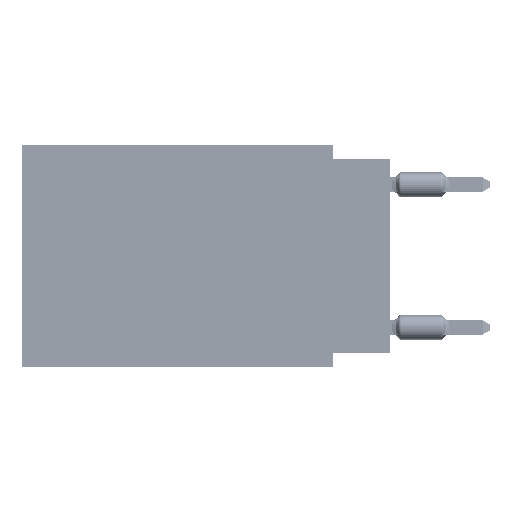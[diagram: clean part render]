
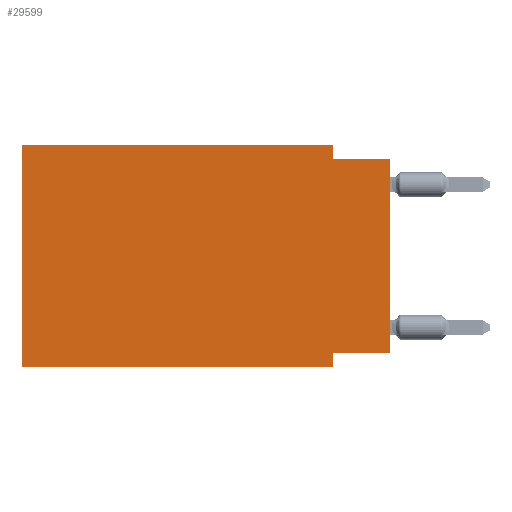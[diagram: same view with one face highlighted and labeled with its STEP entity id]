
A CAD part, left-side view. The second image highlights one B-rep face of the part: STEP entity #29599.
In plain terms, the highlighted planar face has unit normal (-1, 0, 0).
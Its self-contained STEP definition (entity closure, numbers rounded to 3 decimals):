
#4770 = CARTESIAN_POINT ( 'NONE',  ( 0., 16.383, 0. ) ) ;
#7644 = EDGE_CURVE ( 'NONE', #35480, #17729, #47735, .T. ) ;
#8155 = ORIENTED_EDGE ( 'NONE', *, *, #63120, .F. ) ;
#8812 = VERTEX_POINT ( 'NONE', #18402 ) ;
#9850 = LINE ( 'NONE', #53430, #20157 ) ;
#10892 = ORIENTED_EDGE ( 'NONE', *, *, #14784, .F. ) ;
#11123 = EDGE_CURVE ( 'NONE', #54508, #53946, #21433, .T. ) ;
#11404 = VERTEX_POINT ( 'NONE', #20290 ) ;
#12124 = VECTOR ( 'NONE', #36971, 1000. ) ;
#14080 = CARTESIAN_POINT ( 'NONE',  ( 0., 0., -0.635 ) ) ;
#14484 = VECTOR ( 'NONE', #26203, 1000. ) ;
#14494 = CARTESIAN_POINT ( 'NONE',  ( 0., 2.54, 0. ) ) ;
#14784 = EDGE_CURVE ( 'NONE', #8812, #11404, #59131, .T. ) ;
#14804 = EDGE_CURVE ( 'NONE', #54508, #35480, #9850, .T. ) ;
#15224 = CARTESIAN_POINT ( 'NONE',  ( 0., 2.54, -9.906 ) ) ;
#17729 = VERTEX_POINT ( 'NONE', #26508 ) ;
#18362 = ORIENTED_EDGE ( 'NONE', *, *, #11123, .T. ) ;
#18402 = CARTESIAN_POINT ( 'NONE',  ( 0., 16.383, -9.906 ) ) ;
#20157 = VECTOR ( 'NONE', #31636, 1000. ) ;
#20290 = CARTESIAN_POINT ( 'NONE',  ( 0., 16.383, 0. ) ) ;
#21433 = LINE ( 'NONE', #48565, #27899 ) ;
#22140 = ORIENTED_EDGE ( 'NONE', *, *, #40206, .F. ) ;
#25946 = CARTESIAN_POINT ( 'NONE',  ( 0., 16.383, 0. ) ) ;
#26121 = ORIENTED_EDGE ( 'NONE', *, *, #36584, .T. ) ;
#26203 = DIRECTION ( 'NONE',  ( 0., -1., 0. ) ) ;
#26508 = CARTESIAN_POINT ( 'NONE',  ( 0., 2.54, -9.906 ) ) ;
#27682 = VERTEX_POINT ( 'NONE', #36505 ) ;
#27688 = EDGE_LOOP ( 'NONE', ( #18362, #22140, #30568, #8155, #10892, #26121, #29860, #68881 ) ) ;
#27899 = VECTOR ( 'NONE', #44600, 1000. ) ;
#28751 = CARTESIAN_POINT ( 'NONE',  ( 0., 16.383, 0. ) ) ;
#29599 = ADVANCED_FACE ( 'NONE', ( #58359 ), #42277, .F. ) ;
#29860 = ORIENTED_EDGE ( 'NONE', *, *, #7644, .F. ) ;
#30568 = ORIENTED_EDGE ( 'NONE', *, *, #65456, .F. ) ;
#31574 = DIRECTION ( 'NONE',  ( 0., 0., -1. ) ) ;
#31636 = DIRECTION ( 'NONE',  ( 0., 1., 0. ) ) ;
#34119 = LINE ( 'NONE', #28751, #69391 ) ;
#34537 = AXIS2_PLACEMENT_3D ( 'NONE', #4770, #58721, #31574 ) ;
#35250 = CARTESIAN_POINT ( 'NONE',  ( 0., 2.54, 0. ) ) ;
#35480 = VERTEX_POINT ( 'NONE', #49610 ) ;
#35752 = CARTESIAN_POINT ( 'NONE',  ( 0., 0., -0.635 ) ) ;
#36505 = CARTESIAN_POINT ( 'NONE',  ( 0., 2.54, -0.635 ) ) ;
#36526 = CARTESIAN_POINT ( 'NONE',  ( 0., 16.383, -9.906 ) ) ;
#36584 = EDGE_CURVE ( 'NONE', #8812, #17729, #47961, .T. ) ;
#36971 = DIRECTION ( 'NONE',  ( 0., 0., 1. ) ) ;
#39588 = VERTEX_POINT ( 'NONE', #35250 ) ;
#40206 = EDGE_CURVE ( 'NONE', #27682, #53946, #63008, .T. ) ;
#40913 = LINE ( 'NONE', #14494, #52335 ) ;
#41934 = DIRECTION ( 'NONE',  ( 0., -1., 0. ) ) ;
#42277 = PLANE ( 'NONE',  #34537 ) ;
#44600 = DIRECTION ( 'NONE',  ( 0., 0., 1. ) ) ;
#47735 = LINE ( 'NONE', #15224, #62176 ) ;
#47961 = LINE ( 'NONE', #36526, #14484 ) ;
#48565 = CARTESIAN_POINT ( 'NONE',  ( 0., 0., 0. ) ) ;
#49610 = CARTESIAN_POINT ( 'NONE',  ( 0., 2.54, -9.271 ) ) ;
#51256 = DIRECTION ( 'NONE',  ( 0., -1., 0. ) ) ;
#52335 = VECTOR ( 'NONE', #62714, 1000. ) ;
#53430 = CARTESIAN_POINT ( 'NONE',  ( 0., 0., -9.271 ) ) ;
#53946 = VERTEX_POINT ( 'NONE', #35752 ) ;
#54508 = VERTEX_POINT ( 'NONE', #59514 ) ;
#56797 = VECTOR ( 'NONE', #41934, 1000. ) ;
#58359 = FACE_OUTER_BOUND ( 'NONE', #27688, .T. ) ;
#58721 = DIRECTION ( 'NONE',  ( 1., 0., 0. ) ) ;
#59131 = LINE ( 'NONE', #25946, #12124 ) ;
#59514 = CARTESIAN_POINT ( 'NONE',  ( 0., 0., -9.271 ) ) ;
#62176 = VECTOR ( 'NONE', #63080, 1000. ) ;
#62714 = DIRECTION ( 'NONE',  ( 0., 0., -1. ) ) ;
#63008 = LINE ( 'NONE', #14080, #56797 ) ;
#63080 = DIRECTION ( 'NONE',  ( 0., 0., -1. ) ) ;
#63120 = EDGE_CURVE ( 'NONE', #11404, #39588, #34119, .T. ) ;
#65456 = EDGE_CURVE ( 'NONE', #39588, #27682, #40913, .T. ) ;
#68881 = ORIENTED_EDGE ( 'NONE', *, *, #14804, .F. ) ;
#69391 = VECTOR ( 'NONE', #51256, 1000. ) ;
